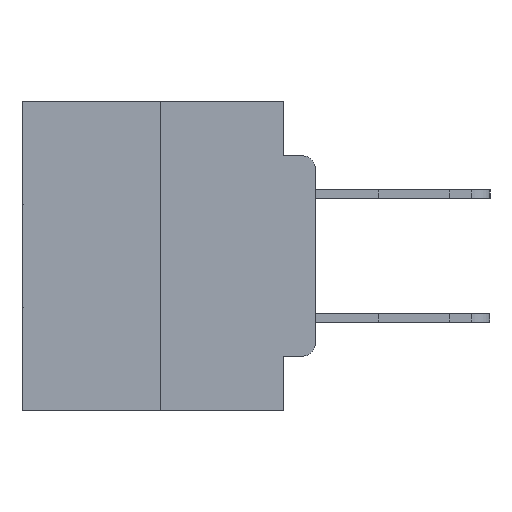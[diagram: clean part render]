
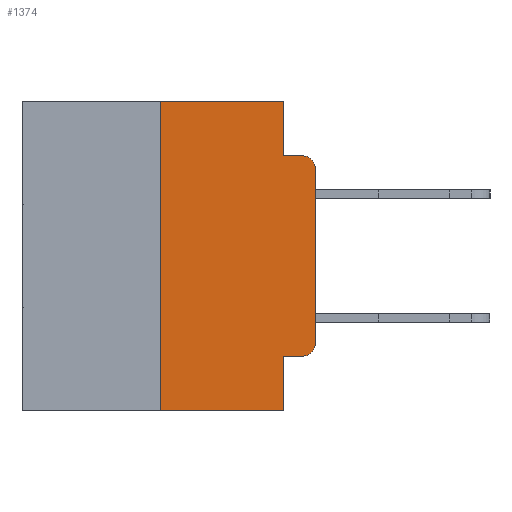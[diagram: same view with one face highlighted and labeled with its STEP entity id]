
A CAD part, left-side view. The second image highlights one B-rep face of the part: STEP entity #1374.
In plain terms, the highlighted planar face has unit normal (-1, 0, 0).
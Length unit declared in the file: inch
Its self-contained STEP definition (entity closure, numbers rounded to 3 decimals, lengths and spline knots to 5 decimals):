
#182 = CARTESIAN_POINT ( 'NONE',  ( 0., 0.473, -0.5 ) ) ;
#213 = LINE ( 'NONE', #27143, #18001 ) ;
#1374 = ADVANCED_FACE ( 'NONE', ( #4672 ), #19975, .F. ) ;
#1699 = ORIENTED_EDGE ( 'NONE', *, *, #12914, .T. ) ;
#1704 = CIRCLE ( 'NONE', #2480, 0.02 ) ;
#2108 = AXIS2_PLACEMENT_3D ( 'NONE', #9611, #24835, #11815 ) ;
#2187 = VERTEX_POINT ( 'NONE', #13085 ) ;
#2465 = CARTESIAN_POINT ( 'NONE',  ( 0., 0.051, 0. ) ) ;
#2480 = AXIS2_PLACEMENT_3D ( 'NONE', #7955, #23253, #10158 ) ;
#2825 = LINE ( 'NONE', #27984, #19764 ) ;
#2872 = VECTOR ( 'NONE', #28135, 39.37008 ) ;
#2873 = CARTESIAN_POINT ( 'NONE',  ( 0., 0.473, 0. ) ) ;
#2954 = EDGE_LOOP ( 'NONE', ( #1699, #24458, #12191, #5620, #8055, #24771, #24123, #18347, #22500, #10173 ) ) ;
#3247 = VERTEX_POINT ( 'NONE', #13665 ) ;
#3920 = DIRECTION ( 'NONE',  ( 0., -1., 0. ) ) ;
#4066 = DIRECTION ( 'NONE',  ( 0., 0., 1. ) ) ;
#4103 = VECTOR ( 'NONE', #26634, 39.37008 ) ;
#4152 = VECTOR ( 'NONE', #17955, 39.37008 ) ;
#4285 = EDGE_CURVE ( 'NONE', #3247, #25376, #213, .T. ) ;
#4490 = CARTESIAN_POINT ( 'NONE',  ( 0., 0.051, 0. ) ) ;
#4672 = FACE_OUTER_BOUND ( 'NONE', #2954, .T. ) ;
#4853 = LINE ( 'NONE', #2465, #4152 ) ;
#4982 = VERTEX_POINT ( 'NONE', #26084 ) ;
#5330 = VECTOR ( 'NONE', #20901, 39.37008 ) ;
#5620 = ORIENTED_EDGE ( 'NONE', *, *, #20107, .F. ) ;
#5690 = CARTESIAN_POINT ( 'NONE',  ( 0., 0.25, 0. ) ) ;
#6208 = VERTEX_POINT ( 'NONE', #22936 ) ;
#7049 = CARTESIAN_POINT ( 'NONE',  ( 0., 0.051, -0.0885 ) ) ;
#7955 = CARTESIAN_POINT ( 'NONE',  ( 0., 0.02, -0.3915 ) ) ;
#7984 = CIRCLE ( 'NONE', #2108, 0.02 ) ;
#8055 = ORIENTED_EDGE ( 'NONE', *, *, #23758, .F. ) ;
#9611 = CARTESIAN_POINT ( 'NONE',  ( 0., 0.02, -0.1085 ) ) ;
#9989 = CARTESIAN_POINT ( 'NONE',  ( 0., 0.051, 0. ) ) ;
#10158 = DIRECTION ( 'NONE',  ( 0., 0., -1. ) ) ;
#10173 = ORIENTED_EDGE ( 'NONE', *, *, #18609, .T. ) ;
#10612 = VERTEX_POINT ( 'NONE', #20640 ) ;
#10814 = CARTESIAN_POINT ( 'NONE',  ( 0., 0.473, 0. ) ) ;
#11349 = VERTEX_POINT ( 'NONE', #14415 ) ;
#11664 = DIRECTION ( 'NONE',  ( 0., 0., -1. ) ) ;
#11815 = DIRECTION ( 'NONE',  ( 0., 0., -1. ) ) ;
#12191 = ORIENTED_EDGE ( 'NONE', *, *, #21706, .F. ) ;
#12388 = VERTEX_POINT ( 'NONE', #4490 ) ;
#12914 = EDGE_CURVE ( 'NONE', #10612, #4982, #2825, .T. ) ;
#13085 = CARTESIAN_POINT ( 'NONE',  ( 0., 0.25, 0. ) ) ;
#13665 = CARTESIAN_POINT ( 'NONE',  ( 0., 0.051, -0.4115 ) ) ;
#13790 = VECTOR ( 'NONE', #20197, 39.37008 ) ;
#14018 = LINE ( 'NONE', #10814, #2872 ) ;
#14415 = CARTESIAN_POINT ( 'NONE',  ( 0., 0.02, -0.0885 ) ) ;
#14614 = CARTESIAN_POINT ( 'NONE',  ( 0., 0.051, -0.5 ) ) ;
#14625 = VERTEX_POINT ( 'NONE', #14614 ) ;
#15153 = LINE ( 'NONE', #182, #13790 ) ;
#15160 = DIRECTION ( 'NONE',  ( 1., 0., 0. ) ) ;
#15478 = VECTOR ( 'NONE', #25351, 39.37008 ) ;
#17070 = LINE ( 'NONE', #9989, #5330 ) ;
#17955 = DIRECTION ( 'NONE',  ( 0., 0., -1. ) ) ;
#18001 = VECTOR ( 'NONE', #3920, 39.37008 ) ;
#18347 = ORIENTED_EDGE ( 'NONE', *, *, #26753, .F. ) ;
#18609 = EDGE_CURVE ( 'NONE', #25376, #10612, #1704, .T. ) ;
#19764 = VECTOR ( 'NONE', #4066, 39.37008 ) ;
#19975 = PLANE ( 'NONE',  #21044 ) ;
#20107 = EDGE_CURVE ( 'NONE', #12388, #6208, #4853, .T. ) ;
#20197 = DIRECTION ( 'NONE',  ( 0., -1., 0. ) ) ;
#20218 = EDGE_CURVE ( 'NONE', #4982, #11349, #7984, .T. ) ;
#20640 = CARTESIAN_POINT ( 'NONE',  ( 0., 0., -0.3915 ) ) ;
#20901 = DIRECTION ( 'NONE',  ( 0., 0., -1. ) ) ;
#21044 = AXIS2_PLACEMENT_3D ( 'NONE', #2873, #15160, #11664 ) ;
#21272 = LINE ( 'NONE', #5690, #15478 ) ;
#21593 = CARTESIAN_POINT ( 'NONE',  ( 0., 0.25, -0.5 ) ) ;
#21706 = EDGE_CURVE ( 'NONE', #6208, #11349, #27304, .T. ) ;
#22093 = VERTEX_POINT ( 'NONE', #21593 ) ;
#22500 = ORIENTED_EDGE ( 'NONE', *, *, #4285, .T. ) ;
#22936 = CARTESIAN_POINT ( 'NONE',  ( 0., 0.051, -0.0885 ) ) ;
#23253 = DIRECTION ( 'NONE',  ( -1., 0., 0. ) ) ;
#23758 = EDGE_CURVE ( 'NONE', #2187, #12388, #14018, .T. ) ;
#24123 = ORIENTED_EDGE ( 'NONE', *, *, #25194, .T. ) ;
#24458 = ORIENTED_EDGE ( 'NONE', *, *, #20218, .T. ) ;
#24771 = ORIENTED_EDGE ( 'NONE', *, *, #25330, .F. ) ;
#24835 = DIRECTION ( 'NONE',  ( -1., 0., 0. ) ) ;
#25194 = EDGE_CURVE ( 'NONE', #22093, #14625, #15153, .T. ) ;
#25330 = EDGE_CURVE ( 'NONE', #22093, #2187, #21272, .T. ) ;
#25351 = DIRECTION ( 'NONE',  ( 0., 0., 1. ) ) ;
#25376 = VERTEX_POINT ( 'NONE', #27591 ) ;
#26084 = CARTESIAN_POINT ( 'NONE',  ( 0., 0., -0.1085 ) ) ;
#26634 = DIRECTION ( 'NONE',  ( 0., -1., 0. ) ) ;
#26753 = EDGE_CURVE ( 'NONE', #3247, #14625, #17070, .T. ) ;
#27143 = CARTESIAN_POINT ( 'NONE',  ( 0., 0.051, -0.4115 ) ) ;
#27304 = LINE ( 'NONE', #7049, #4103 ) ;
#27591 = CARTESIAN_POINT ( 'NONE',  ( 0., 0.02, -0.4115 ) ) ;
#27984 = CARTESIAN_POINT ( 'NONE',  ( 0., 0., 0. ) ) ;
#28135 = DIRECTION ( 'NONE',  ( 0., -1., 0. ) ) ;
